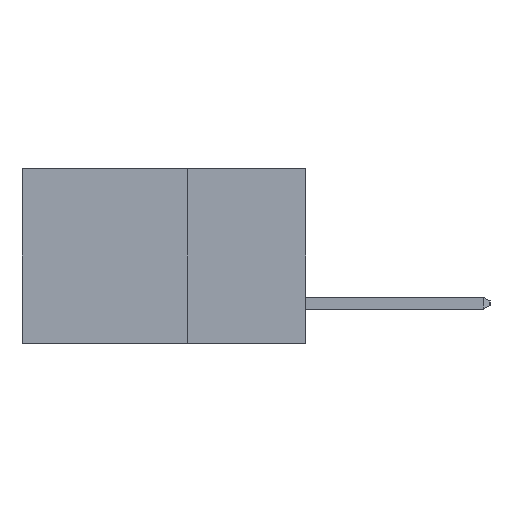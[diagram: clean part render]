
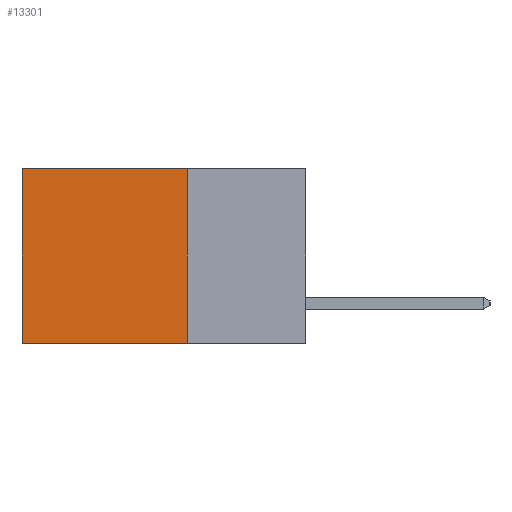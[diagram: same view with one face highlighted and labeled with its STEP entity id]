
A CAD part, left-side view. The second image highlights one B-rep face of the part: STEP entity #13301.
In plain terms, the highlighted planar face has unit normal (-1, 0, 0).
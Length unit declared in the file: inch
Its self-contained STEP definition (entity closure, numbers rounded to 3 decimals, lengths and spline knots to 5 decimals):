
#469 = CARTESIAN_POINT ( 'NONE',  ( 0.298, 0.6, 0. ) ) ;
#2349 = DIRECTION ( 'NONE',  ( 0., 0., -1. ) ) ;
#2642 = VERTEX_POINT ( 'NONE', #24204 ) ;
#3296 = DIRECTION ( 'NONE',  ( 0., 1., 0. ) ) ;
#3343 = FACE_OUTER_BOUND ( 'NONE', #9468, .T. ) ;
#3884 = ORIENTED_EDGE ( 'NONE', *, *, #22757, .T. ) ;
#4074 = EDGE_CURVE ( 'NONE', #5129, #10807, #18298, .T. ) ;
#4892 = CARTESIAN_POINT ( 'NONE',  ( 0.298, 0.25, 0. ) ) ;
#5129 = VERTEX_POINT ( 'NONE', #7998 ) ;
#5806 = ORIENTED_EDGE ( 'NONE', *, *, #11124, .F. ) ;
#5980 = AXIS2_PLACEMENT_3D ( 'NONE', #11120, #24695, #13083 ) ;
#6740 = LINE ( 'NONE', #10941, #10074 ) ;
#6866 = VERTEX_POINT ( 'NONE', #14001 ) ;
#7532 = VECTOR ( 'NONE', #2349, 39.37008 ) ;
#7998 = CARTESIAN_POINT ( 'NONE',  ( 0.298, 0.25, 0. ) ) ;
#9468 = EDGE_LOOP ( 'NONE', ( #3884, #5806, #11513, #23669 ) ) ;
#10074 = VECTOR ( 'NONE', #3296, 39.37008 ) ;
#10807 = VERTEX_POINT ( 'NONE', #15888 ) ;
#10941 = CARTESIAN_POINT ( 'NONE',  ( 0.298, 0.25, -0.37 ) ) ;
#11092 = CARTESIAN_POINT ( 'NONE',  ( 0.298, 0.25, 0. ) ) ;
#11120 = CARTESIAN_POINT ( 'NONE',  ( 0.298, 0.25, 0. ) ) ;
#11124 = EDGE_CURVE ( 'NONE', #10807, #2642, #6740, .T. ) ;
#11513 = ORIENTED_EDGE ( 'NONE', *, *, #4074, .F. ) ;
#13083 = DIRECTION ( 'NONE',  ( 0., 0., -1. ) ) ;
#13301 = ADVANCED_FACE ( 'NONE', ( #3343 ), #20778, .F. ) ;
#14001 = CARTESIAN_POINT ( 'NONE',  ( 0.298, 0.6, 0. ) ) ;
#14509 = DIRECTION ( 'NONE',  ( 0., 1., 0. ) ) ;
#15888 = CARTESIAN_POINT ( 'NONE',  ( 0.298, 0.25, -0.37 ) ) ;
#15963 = EDGE_CURVE ( 'NONE', #5129, #6866, #16558, .T. ) ;
#16558 = LINE ( 'NONE', #4892, #21687 ) ;
#18298 = LINE ( 'NONE', #11092, #22240 ) ;
#20778 = PLANE ( 'NONE',  #5980 ) ;
#21687 = VECTOR ( 'NONE', #14509, 39.37008 ) ;
#22240 = VECTOR ( 'NONE', #24227, 39.37008 ) ;
#22415 = LINE ( 'NONE', #469, #7532 ) ;
#22757 = EDGE_CURVE ( 'NONE', #6866, #2642, #22415, .T. ) ;
#23669 = ORIENTED_EDGE ( 'NONE', *, *, #15963, .T. ) ;
#24204 = CARTESIAN_POINT ( 'NONE',  ( 0.298, 0.6, -0.37 ) ) ;
#24227 = DIRECTION ( 'NONE',  ( 0., 0., -1. ) ) ;
#24695 = DIRECTION ( 'NONE',  ( 1., 0., 0. ) ) ;
